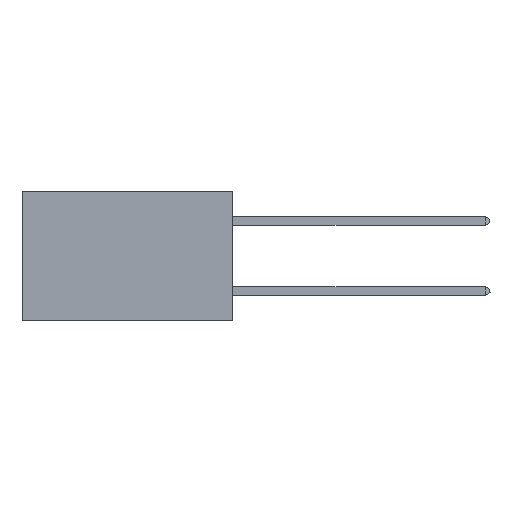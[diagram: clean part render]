
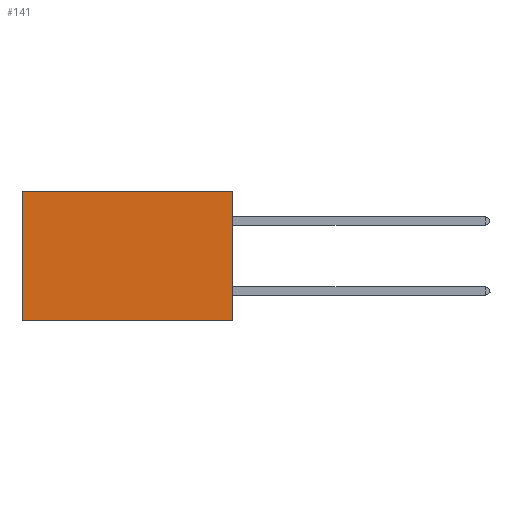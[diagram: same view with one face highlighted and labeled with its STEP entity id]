
A CAD part, left-side view. The second image highlights one B-rep face of the part: STEP entity #141.
In plain terms, the highlighted planar face has unit normal (-1, 0, 0).
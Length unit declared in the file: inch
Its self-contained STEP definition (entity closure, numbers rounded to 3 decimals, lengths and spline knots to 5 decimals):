
#141 = ADVANCED_FACE ( 'NONE', ( #9857 ), #8805, .F. ) ;
#371 = CARTESIAN_POINT ( 'NONE',  ( 0.2875, 0., 0. ) ) ;
#409 = CARTESIAN_POINT ( 'NONE',  ( 0.2875, 0., 0. ) ) ;
#435 = CARTESIAN_POINT ( 'NONE',  ( 0.2875, 0., 0. ) ) ;
#789 = CARTESIAN_POINT ( 'NONE',  ( 0.2875, 0.6, 0. ) ) ;
#1791 = CARTESIAN_POINT ( 'NONE',  ( 0.2875, 0., 0. ) ) ;
#1932 = VERTEX_POINT ( 'NONE', #9894 ) ;
#3314 = ORIENTED_EDGE ( 'NONE', *, *, #9237, .T. ) ;
#4345 = CARTESIAN_POINT ( 'NONE',  ( 0.2875, 0.6, 0. ) ) ;
#5314 = EDGE_LOOP ( 'NONE', ( #3314, #14460, #24564, #19690 ) ) ;
#5367 = VECTOR ( 'NONE', #10975, 39.37008 ) ;
#6161 = DIRECTION ( 'NONE',  ( 0., 1., 0. ) ) ;
#7855 = AXIS2_PLACEMENT_3D ( 'NONE', #371, #13796, #19006 ) ;
#8290 = DIRECTION ( 'NONE',  ( 0., 0., -1. ) ) ;
#8805 = PLANE ( 'NONE',  #7855 ) ;
#9237 = EDGE_CURVE ( 'NONE', #26631, #1932, #31334, .T. ) ;
#9857 = FACE_OUTER_BOUND ( 'NONE', #5314, .T. ) ;
#9894 = CARTESIAN_POINT ( 'NONE',  ( 0.2875, 0.6, -0.37 ) ) ;
#10975 = DIRECTION ( 'NONE',  ( 0., 1., 0. ) ) ;
#12964 = EDGE_CURVE ( 'NONE', #24218, #1932, #22004, .T. ) ;
#13796 = DIRECTION ( 'NONE',  ( 1., 0., 0. ) ) ;
#14460 = ORIENTED_EDGE ( 'NONE', *, *, #12964, .F. ) ;
#15146 = DIRECTION ( 'NONE',  ( 0., 0., -1. ) ) ;
#17280 = LINE ( 'NONE', #435, #26887 ) ;
#19006 = DIRECTION ( 'NONE',  ( 0., 0., -1. ) ) ;
#19690 = ORIENTED_EDGE ( 'NONE', *, *, #29153, .T. ) ;
#20849 = VERTEX_POINT ( 'NONE', #1791 ) ;
#21215 = CARTESIAN_POINT ( 'NONE',  ( 0.2875, 0., -0.37 ) ) ;
#22004 = LINE ( 'NONE', #21215, #5367 ) ;
#24218 = VERTEX_POINT ( 'NONE', #32405 ) ;
#24564 = ORIENTED_EDGE ( 'NONE', *, *, #25397, .F. ) ;
#25225 = LINE ( 'NONE', #409, #33947 ) ;
#25397 = EDGE_CURVE ( 'NONE', #20849, #24218, #17280, .T. ) ;
#26631 = VERTEX_POINT ( 'NONE', #789 ) ;
#26887 = VECTOR ( 'NONE', #8290, 39.37008 ) ;
#29153 = EDGE_CURVE ( 'NONE', #20849, #26631, #25225, .T. ) ;
#30942 = VECTOR ( 'NONE', #15146, 39.37008 ) ;
#31334 = LINE ( 'NONE', #4345, #30942 ) ;
#32405 = CARTESIAN_POINT ( 'NONE',  ( 0.2875, 0., -0.37 ) ) ;
#33947 = VECTOR ( 'NONE', #6161, 39.37008 ) ;
